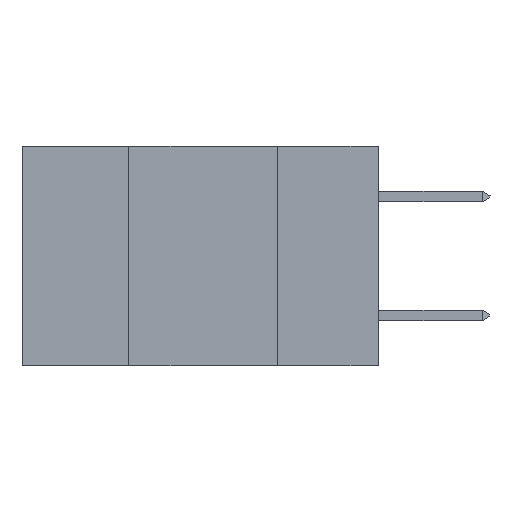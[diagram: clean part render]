
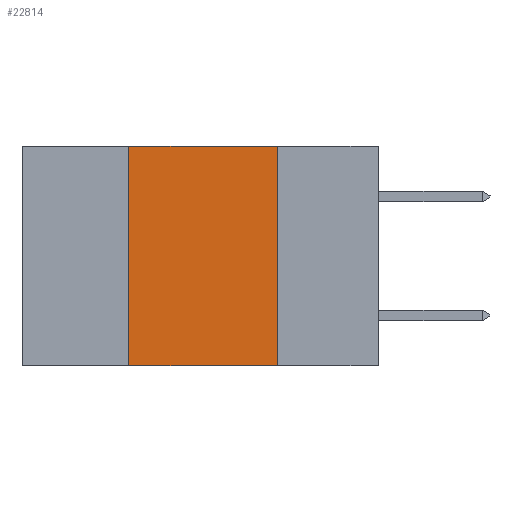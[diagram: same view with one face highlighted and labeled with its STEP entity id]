
A CAD part, left-side view. The second image highlights one B-rep face of the part: STEP entity #22814.
In plain terms, the highlighted planar face has unit normal (-1, 0, 0).
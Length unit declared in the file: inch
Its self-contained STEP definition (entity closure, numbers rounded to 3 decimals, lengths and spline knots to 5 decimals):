
#1255 = ORIENTED_EDGE ( 'NONE', *, *, #25821, .F. ) ;
#1851 = PLANE ( 'NONE',  #11889 ) ;
#2882 = ORIENTED_EDGE ( 'NONE', *, *, #10256, .F. ) ;
#3877 = FACE_OUTER_BOUND ( 'NONE', #10740, .T. ) ;
#5284 = CARTESIAN_POINT ( 'NONE',  ( 0., 0.42, -0.37 ) ) ;
#5493 = DIRECTION ( 'NONE',  ( 0., -1., 0. ) ) ;
#6352 = CARTESIAN_POINT ( 'NONE',  ( 0., 0.6, -0.37 ) ) ;
#7594 = VECTOR ( 'NONE', #16516, 39.37008 ) ;
#8193 = CARTESIAN_POINT ( 'NONE',  ( 0., 0.6, 0. ) ) ;
#8246 = VERTEX_POINT ( 'NONE', #11684 ) ;
#8688 = VERTEX_POINT ( 'NONE', #5284 ) ;
#10256 = EDGE_CURVE ( 'NONE', #19342, #8246, #17836, .T. ) ;
#10324 = CARTESIAN_POINT ( 'NONE',  ( 0., 0.17, -0.37 ) ) ;
#10531 = EDGE_CURVE ( 'NONE', #8246, #11236, #17289, .T. ) ;
#10740 = EDGE_LOOP ( 'NONE', ( #24115, #2882, #1255, #22955 ) ) ;
#11236 = VERTEX_POINT ( 'NONE', #10324 ) ;
#11684 = CARTESIAN_POINT ( 'NONE',  ( 0., 0.17, 0. ) ) ;
#11889 = AXIS2_PLACEMENT_3D ( 'NONE', #8193, #24644, #24364 ) ;
#12065 = LINE ( 'NONE', #24695, #24075 ) ;
#14362 = DIRECTION ( 'NONE',  ( 0., 0., 1. ) ) ;
#15103 = VECTOR ( 'NONE', #5493, 39.37008 ) ;
#16516 = DIRECTION ( 'NONE',  ( 0., -1., 0. ) ) ;
#17289 = LINE ( 'NONE', #20954, #23792 ) ;
#17836 = LINE ( 'NONE', #24095, #15103 ) ;
#19342 = VERTEX_POINT ( 'NONE', #23037 ) ;
#20954 = CARTESIAN_POINT ( 'NONE',  ( 0., 0.17, -0.37 ) ) ;
#22758 = LINE ( 'NONE', #6352, #7594 ) ;
#22814 = ADVANCED_FACE ( 'NONE', ( #3877 ), #1851, .F. ) ;
#22955 = ORIENTED_EDGE ( 'NONE', *, *, #25705, .T. ) ;
#23037 = CARTESIAN_POINT ( 'NONE',  ( 0., 0.42, 0. ) ) ;
#23792 = VECTOR ( 'NONE', #25440, 39.37008 ) ;
#24075 = VECTOR ( 'NONE', #14362, 39.37008 ) ;
#24095 = CARTESIAN_POINT ( 'NONE',  ( 0., 0.6, 0. ) ) ;
#24115 = ORIENTED_EDGE ( 'NONE', *, *, #10531, .F. ) ;
#24364 = DIRECTION ( 'NONE',  ( 0., 0., -1. ) ) ;
#24644 = DIRECTION ( 'NONE',  ( 1., 0., 0. ) ) ;
#24695 = CARTESIAN_POINT ( 'NONE',  ( 0., 0.42, -0.37 ) ) ;
#25440 = DIRECTION ( 'NONE',  ( 0., 0., -1. ) ) ;
#25705 = EDGE_CURVE ( 'NONE', #8688, #11236, #22758, .T. ) ;
#25821 = EDGE_CURVE ( 'NONE', #8688, #19342, #12065, .T. ) ;
